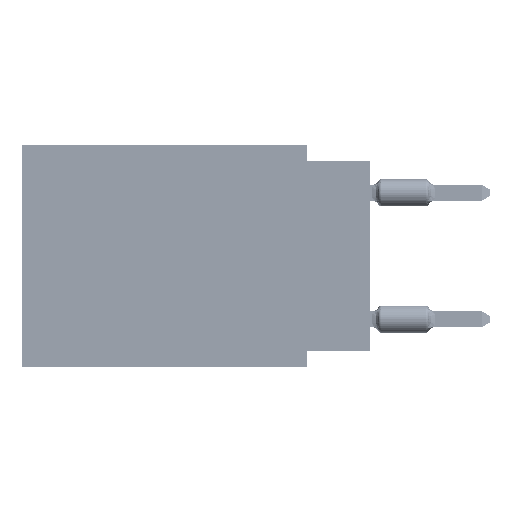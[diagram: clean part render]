
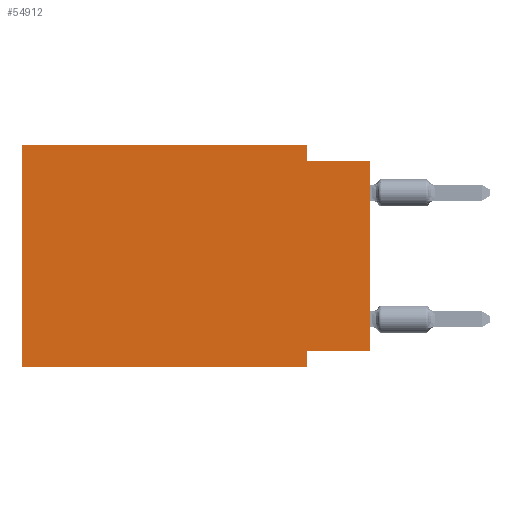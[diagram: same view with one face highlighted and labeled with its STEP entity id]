
A CAD part, left-side view. The second image highlights one B-rep face of the part: STEP entity #54912.
In plain terms, the highlighted planar face has unit normal (-1, 0, 0).
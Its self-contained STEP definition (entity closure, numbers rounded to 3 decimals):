
#1215 = VECTOR ( 'NONE', #11109, 1000. ) ;
#2094 = ORIENTED_EDGE ( 'NONE', *, *, #11684, .T. ) ;
#3118 = CARTESIAN_POINT ( 'NONE',  ( 0., 2.54, 0. ) ) ;
#5392 = VECTOR ( 'NONE', #57518, 1000. ) ;
#6804 = EDGE_CURVE ( 'NONE', #33111, #48596, #20144, .T. ) ;
#6818 = EDGE_CURVE ( 'NONE', #48596, #56087, #12433, .T. ) ;
#7024 = ORIENTED_EDGE ( 'NONE', *, *, #68783, .F. ) ;
#7479 = CARTESIAN_POINT ( 'NONE',  ( 0., 13.97, 0. ) ) ;
#8188 = EDGE_CURVE ( 'NONE', #47710, #45000, #42529, .T. ) ;
#10359 = LINE ( 'NONE', #3118, #82318 ) ;
#11066 = PLANE ( 'NONE',  #79372 ) ;
#11109 = DIRECTION ( 'NONE',  ( 0., -1., 0. ) ) ;
#11529 = DIRECTION ( 'NONE',  ( 0., 0., 1. ) ) ;
#11684 = EDGE_CURVE ( 'NONE', #33111, #48741, #67277, .T. ) ;
#12433 = LINE ( 'NONE', #46881, #68795 ) ;
#12684 = ORIENTED_EDGE ( 'NONE', *, *, #48079, .F. ) ;
#13358 = LINE ( 'NONE', #61392, #62966 ) ;
#15853 = LINE ( 'NONE', #30329, #5392 ) ;
#18030 = CARTESIAN_POINT ( 'NONE',  ( 0., 2.54, -8.89 ) ) ;
#18733 = ORIENTED_EDGE ( 'NONE', *, *, #35767, .T. ) ;
#19707 = CARTESIAN_POINT ( 'NONE',  ( 0., 2.54, -0.635 ) ) ;
#20144 = LINE ( 'NONE', #74511, #32536 ) ;
#20612 = DIRECTION ( 'NONE',  ( 0., -1., 0. ) ) ;
#22752 = CARTESIAN_POINT ( 'NONE',  ( 0., 13.97, -8.89 ) ) ;
#25973 = ORIENTED_EDGE ( 'NONE', *, *, #6804, .F. ) ;
#26190 = CARTESIAN_POINT ( 'NONE',  ( 0., 2.54, 0. ) ) ;
#30329 = CARTESIAN_POINT ( 'NONE',  ( 0., 0., 0. ) ) ;
#31627 = LINE ( 'NONE', #18030, #84392 ) ;
#32536 = VECTOR ( 'NONE', #11529, 1000. ) ;
#32787 = CARTESIAN_POINT ( 'NONE',  ( 0., 13.97, 0. ) ) ;
#33111 = VERTEX_POINT ( 'NONE', #22752 ) ;
#35767 = EDGE_CURVE ( 'NONE', #47710, #65830, #15853, .T. ) ;
#42529 = LINE ( 'NONE', #70604, #53037 ) ;
#45000 = VERTEX_POINT ( 'NONE', #78366 ) ;
#46331 = CARTESIAN_POINT ( 'NONE',  ( 0., 0., -8.255 ) ) ;
#46881 = CARTESIAN_POINT ( 'NONE',  ( 0., 13.97, 0. ) ) ;
#47710 = VERTEX_POINT ( 'NONE', #46331 ) ;
#48079 = EDGE_CURVE ( 'NONE', #45000, #48741, #31627, .T. ) ;
#48596 = VERTEX_POINT ( 'NONE', #7479 ) ;
#48741 = VERTEX_POINT ( 'NONE', #70887 ) ;
#48874 = DIRECTION ( 'NONE',  ( 0., 1., 0. ) ) ;
#53037 = VECTOR ( 'NONE', #48874, 1000. ) ;
#53354 = DIRECTION ( 'NONE',  ( 0., 0., -1. ) ) ;
#54912 = ADVANCED_FACE ( 'NONE', ( #73155 ), #11066, .F. ) ;
#56087 = VERTEX_POINT ( 'NONE', #26190 ) ;
#57518 = DIRECTION ( 'NONE',  ( 0., 0., 1. ) ) ;
#59560 = CARTESIAN_POINT ( 'NONE',  ( 0., 13.97, -8.89 ) ) ;
#59898 = VERTEX_POINT ( 'NONE', #19707 ) ;
#59966 = DIRECTION ( 'NONE',  ( 0., 0., -1. ) ) ;
#61392 = CARTESIAN_POINT ( 'NONE',  ( 0., 0., -0.635 ) ) ;
#62966 = VECTOR ( 'NONE', #20612, 1000. ) ;
#65203 = EDGE_CURVE ( 'NONE', #59898, #65830, #13358, .T. ) ;
#65830 = VERTEX_POINT ( 'NONE', #77902 ) ;
#66166 = EDGE_LOOP ( 'NONE', ( #18733, #77750, #7024, #81855, #25973, #2094, #12684, #83500 ) ) ;
#67277 = LINE ( 'NONE', #59560, #1215 ) ;
#68783 = EDGE_CURVE ( 'NONE', #56087, #59898, #10359, .T. ) ;
#68795 = VECTOR ( 'NONE', #75413, 1000. ) ;
#70604 = CARTESIAN_POINT ( 'NONE',  ( 0., 0., -8.255 ) ) ;
#70887 = CARTESIAN_POINT ( 'NONE',  ( 0., 2.54, -8.89 ) ) ;
#73155 = FACE_OUTER_BOUND ( 'NONE', #66166, .T. ) ;
#74511 = CARTESIAN_POINT ( 'NONE',  ( 0., 13.97, 0. ) ) ;
#75413 = DIRECTION ( 'NONE',  ( 0., -1., 0. ) ) ;
#77750 = ORIENTED_EDGE ( 'NONE', *, *, #65203, .F. ) ;
#77902 = CARTESIAN_POINT ( 'NONE',  ( 0., 0., -0.635 ) ) ;
#78366 = CARTESIAN_POINT ( 'NONE',  ( 0., 2.54, -8.255 ) ) ;
#79228 = DIRECTION ( 'NONE',  ( 0., 0., -1. ) ) ;
#79372 = AXIS2_PLACEMENT_3D ( 'NONE', #32787, #86741, #59966 ) ;
#81855 = ORIENTED_EDGE ( 'NONE', *, *, #6818, .F. ) ;
#82318 = VECTOR ( 'NONE', #79228, 1000. ) ;
#83500 = ORIENTED_EDGE ( 'NONE', *, *, #8188, .F. ) ;
#84392 = VECTOR ( 'NONE', #53354, 1000. ) ;
#86741 = DIRECTION ( 'NONE',  ( 1., 0., 0. ) ) ;
